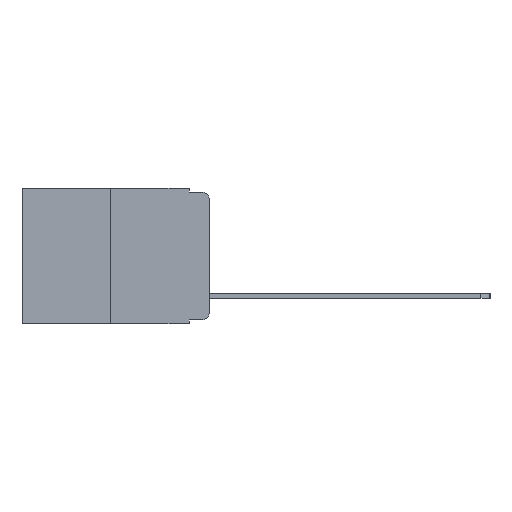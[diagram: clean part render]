
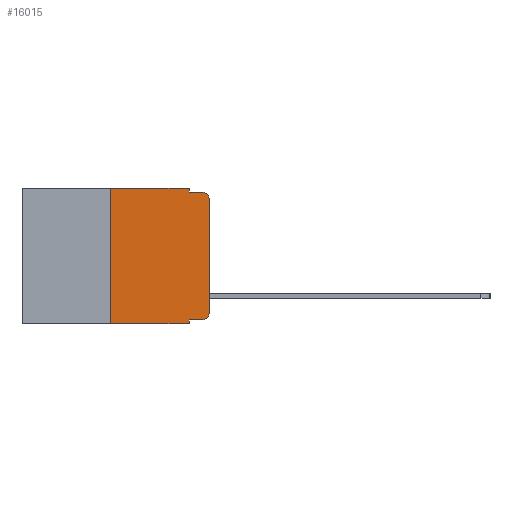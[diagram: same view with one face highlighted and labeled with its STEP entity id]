
A CAD part, left-side view. The second image highlights one B-rep face of the part: STEP entity #16015.
In plain terms, the highlighted planar face has unit normal (-1, 0, 0).
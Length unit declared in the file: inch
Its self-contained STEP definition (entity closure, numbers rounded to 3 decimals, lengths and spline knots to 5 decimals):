
#28 = EDGE_CURVE ( 'NONE', #7816, #5397, #14773, .T. ) ;
#897 = AXIS2_PLACEMENT_3D ( 'NONE', #12601, #19574, #9099 ) ;
#990 = EDGE_LOOP ( 'NONE', ( #8572, #17904, #18446, #1134, #15487, #8859, #5209, #15239, #15767, #2009 ) ) ;
#1134 = ORIENTED_EDGE ( 'NONE', *, *, #17169, .F. ) ;
#1146 = VECTOR ( 'NONE', #14181, 39.37008 ) ;
#1528 = VECTOR ( 'NONE', #17548, 39.37008 ) ;
#2009 = ORIENTED_EDGE ( 'NONE', *, *, #8909, .T. ) ;
#2820 = VECTOR ( 'NONE', #8466, 39.37008 ) ;
#3775 = CARTESIAN_POINT ( 'NONE',  ( 0., 0.02, -0.313 ) ) ;
#4160 = DIRECTION ( 'NONE',  ( 0., 0., 1. ) ) ;
#5209 = ORIENTED_EDGE ( 'NONE', *, *, #7589, .T. ) ;
#5288 = VECTOR ( 'NONE', #9576, 39.37008 ) ;
#5397 = VERTEX_POINT ( 'NONE', #6896 ) ;
#5654 = DIRECTION ( 'NONE',  ( 0., 0., -1. ) ) ;
#6034 = DIRECTION ( 'NONE',  ( 0., -1., 0. ) ) ;
#6074 = CARTESIAN_POINT ( 'NONE',  ( 0., 0.25, -0.343 ) ) ;
#6081 = LINE ( 'NONE', #10608, #1146 ) ;
#6353 = CARTESIAN_POINT ( 'NONE',  ( 0., 0.02, -0.01 ) ) ;
#6687 = DIRECTION ( 'NONE',  ( -1., 0., 0. ) ) ;
#6693 = CARTESIAN_POINT ( 'NONE',  ( 0., 0.051, -0.01 ) ) ;
#6896 = CARTESIAN_POINT ( 'NONE',  ( 0., 0.051, 0. ) ) ;
#7010 = LINE ( 'NONE', #15732, #1528 ) ;
#7331 = PLANE ( 'NONE',  #897 ) ;
#7432 = AXIS2_PLACEMENT_3D ( 'NONE', #3775, #16235, #5654 ) ;
#7565 = VERTEX_POINT ( 'NONE', #6353 ) ;
#7589 = EDGE_CURVE ( 'NONE', #15281, #9150, #21996, .T. ) ;
#7816 = VERTEX_POINT ( 'NONE', #8821 ) ;
#8183 = CARTESIAN_POINT ( 'NONE',  ( 0., 0., -0.313 ) ) ;
#8211 = VERTEX_POINT ( 'NONE', #13387 ) ;
#8466 = DIRECTION ( 'NONE',  ( 0., -1., 0. ) ) ;
#8572 = ORIENTED_EDGE ( 'NONE', *, *, #21749, .T. ) ;
#8821 = CARTESIAN_POINT ( 'NONE',  ( 0., 0.25, 0. ) ) ;
#8859 = ORIENTED_EDGE ( 'NONE', *, *, #14862, .F. ) ;
#8909 = EDGE_CURVE ( 'NONE', #8211, #10817, #12741, .T. ) ;
#9099 = DIRECTION ( 'NONE',  ( 0., 0., -1. ) ) ;
#9150 = VERTEX_POINT ( 'NONE', #18567 ) ;
#9161 = VECTOR ( 'NONE', #20735, 39.37008 ) ;
#9304 = VERTEX_POINT ( 'NONE', #10181 ) ;
#9503 = VECTOR ( 'NONE', #6034, 39.37008 ) ;
#9576 = DIRECTION ( 'NONE',  ( 0., -1., 0. ) ) ;
#10031 = VECTOR ( 'NONE', #4160, 39.37008 ) ;
#10181 = CARTESIAN_POINT ( 'NONE',  ( 0., 0.051, -0.333 ) ) ;
#10608 = CARTESIAN_POINT ( 'NONE',  ( 0., 0.051, 0. ) ) ;
#10817 = VERTEX_POINT ( 'NONE', #8183 ) ;
#11292 = EDGE_CURVE ( 'NONE', #9304, #8211, #15307, .T. ) ;
#11704 = CARTESIAN_POINT ( 'NONE',  ( 0., 0.473, -0.343 ) ) ;
#12601 = CARTESIAN_POINT ( 'NONE',  ( 0., 0.473, 0. ) ) ;
#12741 = CIRCLE ( 'NONE', #7432, 0.02 ) ;
#12924 = CARTESIAN_POINT ( 'NONE',  ( 0., 0.051, -0.01 ) ) ;
#13387 = CARTESIAN_POINT ( 'NONE',  ( 0., 0.02, -0.333 ) ) ;
#13681 = EDGE_CURVE ( 'NONE', #9304, #9150, #7010, .T. ) ;
#13685 = AXIS2_PLACEMENT_3D ( 'NONE', #17235, #6687, #18952 ) ;
#13789 = CARTESIAN_POINT ( 'NONE',  ( 0., 0.25, 0. ) ) ;
#14181 = DIRECTION ( 'NONE',  ( 0., 0., -1. ) ) ;
#14773 = LINE ( 'NONE', #21777, #9503 ) ;
#14862 = EDGE_CURVE ( 'NONE', #15281, #7816, #16488, .T. ) ;
#14863 = CARTESIAN_POINT ( 'NONE',  ( 0., 0., 0. ) ) ;
#15239 = ORIENTED_EDGE ( 'NONE', *, *, #13681, .F. ) ;
#15281 = VERTEX_POINT ( 'NONE', #6074 ) ;
#15307 = LINE ( 'NONE', #16557, #5288 ) ;
#15487 = ORIENTED_EDGE ( 'NONE', *, *, #28, .F. ) ;
#15517 = FACE_OUTER_BOUND ( 'NONE', #990, .T. ) ;
#15732 = CARTESIAN_POINT ( 'NONE',  ( 0., 0.051, 0. ) ) ;
#15767 = ORIENTED_EDGE ( 'NONE', *, *, #11292, .T. ) ;
#16015 = ADVANCED_FACE ( 'NONE', ( #15517 ), #7331, .F. ) ;
#16127 = VERTEX_POINT ( 'NONE', #19782 ) ;
#16191 = CIRCLE ( 'NONE', #13685, 0.02 ) ;
#16235 = DIRECTION ( 'NONE',  ( -1., 0., 0. ) ) ;
#16488 = LINE ( 'NONE', #13789, #9161 ) ;
#16557 = CARTESIAN_POINT ( 'NONE',  ( 0., 0.051, -0.333 ) ) ;
#16931 = DIRECTION ( 'NONE',  ( 0., -1., 0. ) ) ;
#17169 = EDGE_CURVE ( 'NONE', #5397, #17359, #6081, .T. ) ;
#17235 = CARTESIAN_POINT ( 'NONE',  ( 0., 0.02, -0.03 ) ) ;
#17359 = VERTEX_POINT ( 'NONE', #12924 ) ;
#17452 = VECTOR ( 'NONE', #16931, 39.37008 ) ;
#17548 = DIRECTION ( 'NONE',  ( 0., 0., -1. ) ) ;
#17904 = ORIENTED_EDGE ( 'NONE', *, *, #19456, .T. ) ;
#18317 = EDGE_CURVE ( 'NONE', #17359, #7565, #21611, .T. ) ;
#18446 = ORIENTED_EDGE ( 'NONE', *, *, #18317, .F. ) ;
#18567 = CARTESIAN_POINT ( 'NONE',  ( 0., 0.051, -0.343 ) ) ;
#18952 = DIRECTION ( 'NONE',  ( 0., 0., -1. ) ) ;
#19306 = LINE ( 'NONE', #14863, #10031 ) ;
#19456 = EDGE_CURVE ( 'NONE', #16127, #7565, #16191, .T. ) ;
#19574 = DIRECTION ( 'NONE',  ( 1., 0., 0. ) ) ;
#19782 = CARTESIAN_POINT ( 'NONE',  ( 0., 0., -0.03 ) ) ;
#20735 = DIRECTION ( 'NONE',  ( 0., 0., 1. ) ) ;
#21611 = LINE ( 'NONE', #6693, #2820 ) ;
#21749 = EDGE_CURVE ( 'NONE', #10817, #16127, #19306, .T. ) ;
#21777 = CARTESIAN_POINT ( 'NONE',  ( 0., 0.473, 0. ) ) ;
#21996 = LINE ( 'NONE', #11704, #17452 ) ;
